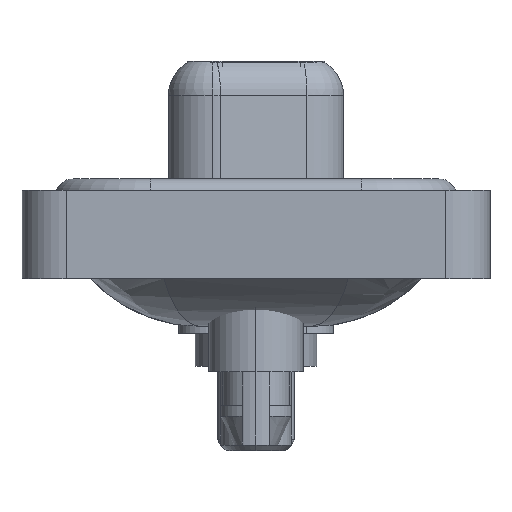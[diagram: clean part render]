
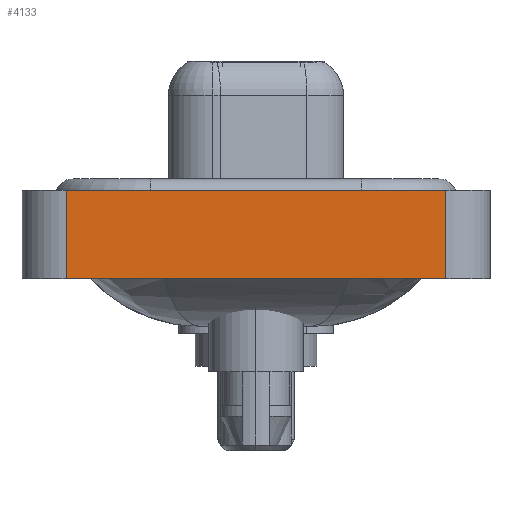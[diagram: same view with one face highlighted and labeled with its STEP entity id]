
A CAD part, left-side view. The second image highlights one B-rep face of the part: STEP entity #4133.
In plain terms, the highlighted planar face has unit normal (-1, 0, 0).
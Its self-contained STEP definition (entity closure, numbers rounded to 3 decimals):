
#435 = CARTESIAN_POINT ( 'NONE',  ( -7.35, -8.55, -3.6 ) ) ;
#1815 = CARTESIAN_POINT ( 'NONE',  ( -7.35, -8.55, 0.4 ) ) ;
#2731 = EDGE_CURVE ( 'NONE', #22810, #5465, #18851, .T. ) ;
#4133 = ADVANCED_FACE ( 'NONE', ( #9801 ), #15141, .T. ) ;
#4444 = VERTEX_POINT ( 'NONE', #1815 ) ;
#4662 = DIRECTION ( 'NONE',  ( 0., 0., 1. ) ) ;
#5000 = VECTOR ( 'NONE', #8181, 1000. ) ;
#5465 = VERTEX_POINT ( 'NONE', #13220 ) ;
#5884 = EDGE_LOOP ( 'NONE', ( #7399, #15967, #18820, #12434 ) ) ;
#7399 = ORIENTED_EDGE ( 'NONE', *, *, #22520, .T. ) ;
#8181 = DIRECTION ( 'NONE',  ( 0., -1., 0. ) ) ;
#8377 = LINE ( 'NONE', #19838, #17514 ) ;
#8455 = VERTEX_POINT ( 'NONE', #15592 ) ;
#8508 = DIRECTION ( 'NONE',  ( -1., 0., 0. ) ) ;
#9801 = FACE_OUTER_BOUND ( 'NONE', #5884, .T. ) ;
#12434 = ORIENTED_EDGE ( 'NONE', *, *, #2731, .T. ) ;
#13220 = CARTESIAN_POINT ( 'NONE',  ( -7.35, -8.55, -3.6 ) ) ;
#13613 = CARTESIAN_POINT ( 'NONE',  ( -7.35, -8.55, -3.6 ) ) ;
#14480 = VECTOR ( 'NONE', #15628, 1000. ) ;
#15141 = PLANE ( 'NONE',  #21592 ) ;
#15592 = CARTESIAN_POINT ( 'NONE',  ( -7.35, 8.55, 0.4 ) ) ;
#15628 = DIRECTION ( 'NONE',  ( 0., 0., 1. ) ) ;
#15967 = ORIENTED_EDGE ( 'NONE', *, *, #21657, .F. ) ;
#16553 = CARTESIAN_POINT ( 'NONE',  ( -7.35, -8.55, -3.6 ) ) ;
#16657 = EDGE_CURVE ( 'NONE', #22810, #8455, #8377, .T. ) ;
#17513 = VECTOR ( 'NONE', #24688, 1000. ) ;
#17514 = VECTOR ( 'NONE', #23765, 1000. ) ;
#18820 = ORIENTED_EDGE ( 'NONE', *, *, #16657, .F. ) ;
#18851 = LINE ( 'NONE', #16553, #17513 ) ;
#19518 = CARTESIAN_POINT ( 'NONE',  ( -7.35, 8.55, -3.6 ) ) ;
#19838 = CARTESIAN_POINT ( 'NONE',  ( -7.35, 8.55, -3.6 ) ) ;
#20037 = CARTESIAN_POINT ( 'NONE',  ( -7.35, -8.55, 0.4 ) ) ;
#21592 = AXIS2_PLACEMENT_3D ( 'NONE', #435, #8508, #4662 ) ;
#21657 = EDGE_CURVE ( 'NONE', #8455, #4444, #23460, .T. ) ;
#22520 = EDGE_CURVE ( 'NONE', #5465, #4444, #25182, .T. ) ;
#22810 = VERTEX_POINT ( 'NONE', #19518 ) ;
#23460 = LINE ( 'NONE', #20037, #5000 ) ;
#23765 = DIRECTION ( 'NONE',  ( 0., 0., 1. ) ) ;
#24688 = DIRECTION ( 'NONE',  ( 0., -1., 0. ) ) ;
#25182 = LINE ( 'NONE', #13613, #14480 ) ;
